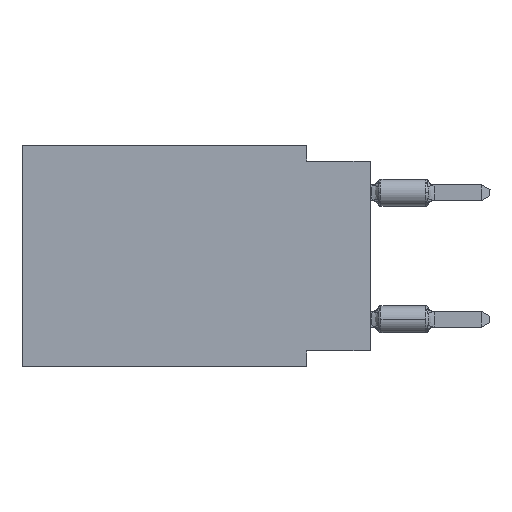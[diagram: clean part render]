
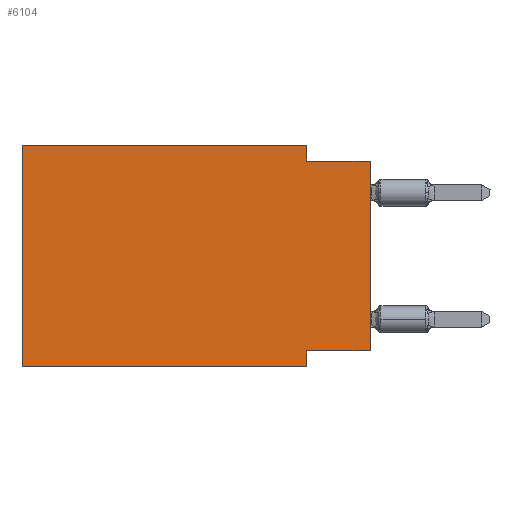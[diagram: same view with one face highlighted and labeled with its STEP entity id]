
A CAD part, left-side view. The second image highlights one B-rep face of the part: STEP entity #6104.
In plain terms, the highlighted planar face has unit normal (-1, 0, 0).
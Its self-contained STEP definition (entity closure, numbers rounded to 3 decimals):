
#1465 = CARTESIAN_POINT ( 'NONE',  ( 0., 2.54, 0. ) ) ;
#1632 = VECTOR ( 'NONE', #24787, 1000. ) ;
#1706 = CARTESIAN_POINT ( 'NONE',  ( 0., 0., -8.255 ) ) ;
#1843 = VECTOR ( 'NONE', #24995, 1000. ) ;
#1895 = ORIENTED_EDGE ( 'NONE', *, *, #35057, .F. ) ;
#2038 = CARTESIAN_POINT ( 'NONE',  ( 0., 2.54, -8.89 ) ) ;
#2205 = LINE ( 'NONE', #2572, #30135 ) ;
#2322 = ORIENTED_EDGE ( 'NONE', *, *, #33919, .F. ) ;
#2572 = CARTESIAN_POINT ( 'NONE',  ( 0., 13.97, 0. ) ) ;
#2730 = VECTOR ( 'NONE', #28187, 1000. ) ;
#4557 = VECTOR ( 'NONE', #5354, 1000. ) ;
#5072 = EDGE_CURVE ( 'NONE', #5442, #34308, #24104, .T. ) ;
#5354 = DIRECTION ( 'NONE',  ( 0., 0., 1. ) ) ;
#5442 = VERTEX_POINT ( 'NONE', #1465 ) ;
#5496 = CARTESIAN_POINT ( 'NONE',  ( 0., 13.97, -8.89 ) ) ;
#6087 = ORIENTED_EDGE ( 'NONE', *, *, #33234, .F. ) ;
#6104 = ADVANCED_FACE ( 'NONE', ( #14643 ), #17010, .F. ) ;
#7337 = CARTESIAN_POINT ( 'NONE',  ( 0., 0., -0.635 ) ) ;
#7445 = VERTEX_POINT ( 'NONE', #7337 ) ;
#7914 = CARTESIAN_POINT ( 'NONE',  ( 0., 0., 0. ) ) ;
#8445 = VERTEX_POINT ( 'NONE', #14540 ) ;
#9127 = VERTEX_POINT ( 'NONE', #35804 ) ;
#11097 = LINE ( 'NONE', #27882, #1632 ) ;
#11217 = EDGE_CURVE ( 'NONE', #16432, #7445, #13907, .T. ) ;
#11527 = CARTESIAN_POINT ( 'NONE',  ( 0., 13.97, -8.89 ) ) ;
#11903 = CARTESIAN_POINT ( 'NONE',  ( 0., 13.97, 0. ) ) ;
#12071 = VERTEX_POINT ( 'NONE', #11527 ) ;
#13142 = DIRECTION ( 'NONE',  ( 0., 0., -1. ) ) ;
#13907 = LINE ( 'NONE', #7914, #4557 ) ;
#14217 = VERTEX_POINT ( 'NONE', #23412 ) ;
#14483 = LINE ( 'NONE', #36008, #34219 ) ;
#14540 = CARTESIAN_POINT ( 'NONE',  ( 0., 2.54, -8.255 ) ) ;
#14643 = FACE_OUTER_BOUND ( 'NONE', #21931, .T. ) ;
#14826 = DIRECTION ( 'NONE',  ( 1., 0., 0. ) ) ;
#15357 = DIRECTION ( 'NONE',  ( 0., 0., -1. ) ) ;
#16432 = VERTEX_POINT ( 'NONE', #1706 ) ;
#17010 = PLANE ( 'NONE',  #30639 ) ;
#17135 = ORIENTED_EDGE ( 'NONE', *, *, #20213, .F. ) ;
#17318 = EDGE_CURVE ( 'NONE', #34308, #7445, #14483, .T. ) ;
#19334 = LINE ( 'NONE', #5496, #1843 ) ;
#19647 = ORIENTED_EDGE ( 'NONE', *, *, #5072, .F. ) ;
#20213 = EDGE_CURVE ( 'NONE', #9127, #5442, #11097, .T. ) ;
#21931 = EDGE_LOOP ( 'NONE', ( #27517, #34083, #19647, #17135, #2322, #27138, #1895, #6087 ) ) ;
#22531 = CARTESIAN_POINT ( 'NONE',  ( 0., 0., -8.255 ) ) ;
#22719 = LINE ( 'NONE', #22531, #2730 ) ;
#23037 = DIRECTION ( 'NONE',  ( 0., 0., -1. ) ) ;
#23412 = CARTESIAN_POINT ( 'NONE',  ( 0., 2.54, -8.89 ) ) ;
#23918 = CARTESIAN_POINT ( 'NONE',  ( 0., 2.54, 0. ) ) ;
#24104 = LINE ( 'NONE', #23918, #33503 ) ;
#24787 = DIRECTION ( 'NONE',  ( 0., -1., 0. ) ) ;
#24995 = DIRECTION ( 'NONE',  ( 0., -1., 0. ) ) ;
#25257 = DIRECTION ( 'NONE',  ( 0., -1., 0. ) ) ;
#27014 = LINE ( 'NONE', #2038, #31923 ) ;
#27138 = ORIENTED_EDGE ( 'NONE', *, *, #30951, .T. ) ;
#27517 = ORIENTED_EDGE ( 'NONE', *, *, #11217, .T. ) ;
#27882 = CARTESIAN_POINT ( 'NONE',  ( 0., 13.97, 0. ) ) ;
#28187 = DIRECTION ( 'NONE',  ( 0., 1., 0. ) ) ;
#30135 = VECTOR ( 'NONE', #33537, 1000. ) ;
#30639 = AXIS2_PLACEMENT_3D ( 'NONE', #11903, #14826, #23037 ) ;
#30951 = EDGE_CURVE ( 'NONE', #12071, #14217, #19334, .T. ) ;
#31923 = VECTOR ( 'NONE', #13142, 1000. ) ;
#33139 = CARTESIAN_POINT ( 'NONE',  ( 0., 2.54, -0.635 ) ) ;
#33234 = EDGE_CURVE ( 'NONE', #16432, #8445, #22719, .T. ) ;
#33503 = VECTOR ( 'NONE', #15357, 1000. ) ;
#33537 = DIRECTION ( 'NONE',  ( 0., 0., 1. ) ) ;
#33919 = EDGE_CURVE ( 'NONE', #12071, #9127, #2205, .T. ) ;
#34083 = ORIENTED_EDGE ( 'NONE', *, *, #17318, .F. ) ;
#34219 = VECTOR ( 'NONE', #25257, 1000. ) ;
#34308 = VERTEX_POINT ( 'NONE', #33139 ) ;
#35057 = EDGE_CURVE ( 'NONE', #8445, #14217, #27014, .T. ) ;
#35804 = CARTESIAN_POINT ( 'NONE',  ( 0., 13.97, 0. ) ) ;
#36008 = CARTESIAN_POINT ( 'NONE',  ( 0., 0., -0.635 ) ) ;
